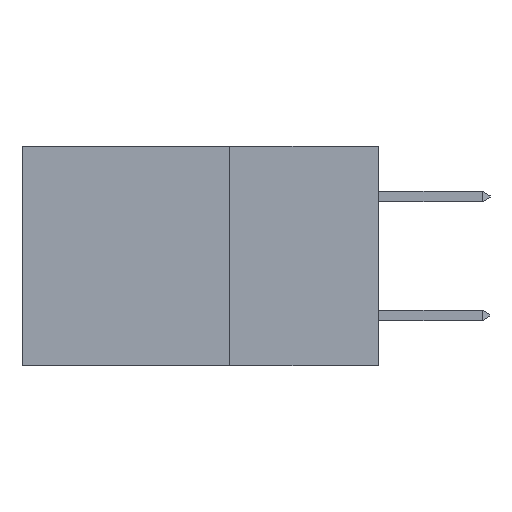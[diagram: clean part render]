
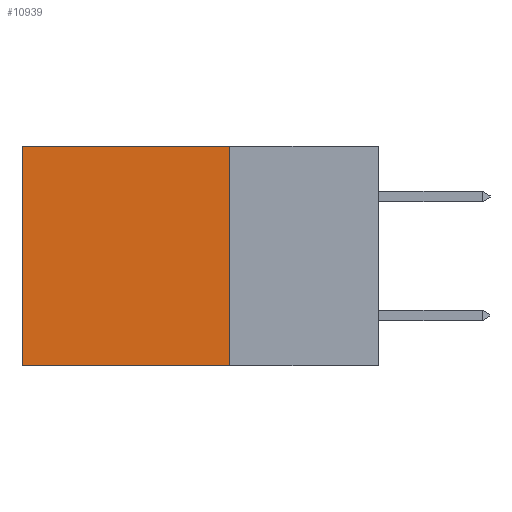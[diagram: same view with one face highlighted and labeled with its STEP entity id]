
A CAD part, left-side view. The second image highlights one B-rep face of the part: STEP entity #10939.
In plain terms, the highlighted planar face has unit normal (-1, 0, 0).
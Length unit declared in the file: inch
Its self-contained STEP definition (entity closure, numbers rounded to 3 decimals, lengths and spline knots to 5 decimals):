
#233 = LINE ( 'NONE', #1178, #3653 ) ;
#1093 = VERTEX_POINT ( 'NONE', #6056 ) ;
#1178 = CARTESIAN_POINT ( 'NONE',  ( 0.298, 0.25, 0. ) ) ;
#1578 = LINE ( 'NONE', #5298, #13793 ) ;
#1865 = EDGE_CURVE ( 'NONE', #1093, #6745, #7434, .T. ) ;
#2025 = CARTESIAN_POINT ( 'NONE',  ( 0.298, 0.6, -0.37 ) ) ;
#3321 = VERTEX_POINT ( 'NONE', #9645 ) ;
#3550 = LINE ( 'NONE', #4644, #9600 ) ;
#3653 = VECTOR ( 'NONE', #7890, 39.37008 ) ;
#3854 = PLANE ( 'NONE',  #5615 ) ;
#4627 = DIRECTION ( 'NONE',  ( 0., 0., -1. ) ) ;
#4644 = CARTESIAN_POINT ( 'NONE',  ( 0.298, 0.6, 0. ) ) ;
#5092 = ORIENTED_EDGE ( 'NONE', *, *, #9891, .T. ) ;
#5298 = CARTESIAN_POINT ( 'NONE',  ( 0.298, 0.25, 0. ) ) ;
#5568 = ORIENTED_EDGE ( 'NONE', *, *, #6805, .T. ) ;
#5615 = AXIS2_PLACEMENT_3D ( 'NONE', #12294, #6246, #14741 ) ;
#5633 = VERTEX_POINT ( 'NONE', #6541 ) ;
#5951 = DIRECTION ( 'NONE',  ( 0., 1., 0. ) ) ;
#6056 = CARTESIAN_POINT ( 'NONE',  ( 0.298, 0.25, -0.37 ) ) ;
#6246 = DIRECTION ( 'NONE',  ( 1., 0., 0. ) ) ;
#6541 = CARTESIAN_POINT ( 'NONE',  ( 0.298, 0.6, 0. ) ) ;
#6745 = VERTEX_POINT ( 'NONE', #2025 ) ;
#6805 = EDGE_CURVE ( 'NONE', #3321, #5633, #233, .T. ) ;
#7058 = VECTOR ( 'NONE', #5951, 39.37008 ) ;
#7434 = LINE ( 'NONE', #13199, #7058 ) ;
#7890 = DIRECTION ( 'NONE',  ( 0., 1., 0. ) ) ;
#8074 = ORIENTED_EDGE ( 'NONE', *, *, #1865, .F. ) ;
#9144 = EDGE_CURVE ( 'NONE', #3321, #1093, #1578, .T. ) ;
#9600 = VECTOR ( 'NONE', #4627, 39.37008 ) ;
#9645 = CARTESIAN_POINT ( 'NONE',  ( 0.298, 0.25, 0. ) ) ;
#9891 = EDGE_CURVE ( 'NONE', #5633, #6745, #3550, .T. ) ;
#10311 = EDGE_LOOP ( 'NONE', ( #5092, #8074, #10549, #5568 ) ) ;
#10549 = ORIENTED_EDGE ( 'NONE', *, *, #9144, .F. ) ;
#10939 = ADVANCED_FACE ( 'NONE', ( #11823 ), #3854, .F. ) ;
#11823 = FACE_OUTER_BOUND ( 'NONE', #10311, .T. ) ;
#12294 = CARTESIAN_POINT ( 'NONE',  ( 0.298, 0.25, 0. ) ) ;
#13199 = CARTESIAN_POINT ( 'NONE',  ( 0.298, 0.25, -0.37 ) ) ;
#13793 = VECTOR ( 'NONE', #15457, 39.37008 ) ;
#14741 = DIRECTION ( 'NONE',  ( 0., 0., -1. ) ) ;
#15457 = DIRECTION ( 'NONE',  ( 0., 0., -1. ) ) ;
